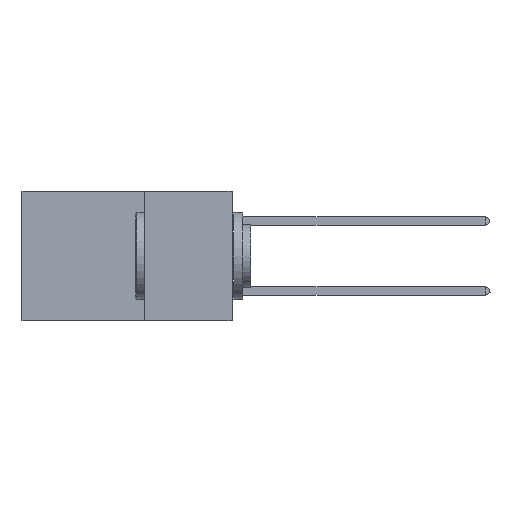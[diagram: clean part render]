
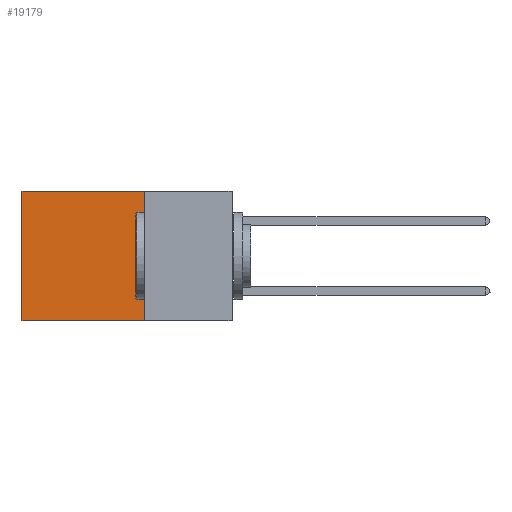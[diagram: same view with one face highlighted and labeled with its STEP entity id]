
A CAD part, left-side view. The second image highlights one B-rep face of the part: STEP entity #19179.
In plain terms, the highlighted planar face has unit normal (-1, 0, 0).
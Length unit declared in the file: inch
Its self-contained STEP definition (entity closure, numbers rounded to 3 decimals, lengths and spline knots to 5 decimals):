
#94 = LINE ( 'NONE', #131, #12554 ) ;
#131 = CARTESIAN_POINT ( 'NONE',  ( 0.2875, 0.25, -0.37 ) ) ;
#309 = VERTEX_POINT ( 'NONE', #5660 ) ;
#1466 = VERTEX_POINT ( 'NONE', #19495 ) ;
#2762 = CARTESIAN_POINT ( 'NONE',  ( 0.2875, 0.25, 0. ) ) ;
#2892 = VECTOR ( 'NONE', #17536, 39.37008 ) ;
#3384 = VERTEX_POINT ( 'NONE', #2762 ) ;
#4023 = CARTESIAN_POINT ( 'NONE',  ( 0.2875, 0.25, 0. ) ) ;
#4850 = CARTESIAN_POINT ( 'NONE',  ( 0.2875, 0.6, 0. ) ) ;
#5660 = CARTESIAN_POINT ( 'NONE',  ( 0.2875, 0.6, -0.37 ) ) ;
#6528 = CARTESIAN_POINT ( 'NONE',  ( 0.2875, 0.25, -0.37 ) ) ;
#7682 = DIRECTION ( 'NONE',  ( 1., 0., 0. ) ) ;
#7691 = AXIS2_PLACEMENT_3D ( 'NONE', #17827, #7682, #21393 ) ;
#7864 = ORIENTED_EDGE ( 'NONE', *, *, #19018, .F. ) ;
#8530 = VECTOR ( 'NONE', #10222, 39.37008 ) ;
#8904 = EDGE_CURVE ( 'NONE', #11808, #309, #94, .T. ) ;
#9281 = FACE_OUTER_BOUND ( 'NONE', #17351, .T. ) ;
#10222 = DIRECTION ( 'NONE',  ( 0., 0., -1. ) ) ;
#10639 = ORIENTED_EDGE ( 'NONE', *, *, #8904, .F. ) ;
#11808 = VERTEX_POINT ( 'NONE', #6528 ) ;
#12255 = ORIENTED_EDGE ( 'NONE', *, *, #18731, .T. ) ;
#12554 = VECTOR ( 'NONE', #18660, 39.37008 ) ;
#13443 = LINE ( 'NONE', #15403, #19291 ) ;
#13878 = ORIENTED_EDGE ( 'NONE', *, *, #14273, .T. ) ;
#14050 = LINE ( 'NONE', #4023, #2892 ) ;
#14273 = EDGE_CURVE ( 'NONE', #3384, #1466, #13443, .T. ) ;
#15403 = CARTESIAN_POINT ( 'NONE',  ( 0.2875, 0.25, 0. ) ) ;
#17100 = DIRECTION ( 'NONE',  ( 0., 1., 0. ) ) ;
#17351 = EDGE_LOOP ( 'NONE', ( #12255, #10639, #7864, #13878 ) ) ;
#17517 = LINE ( 'NONE', #4850, #8530 ) ;
#17536 = DIRECTION ( 'NONE',  ( 0., 0., -1. ) ) ;
#17827 = CARTESIAN_POINT ( 'NONE',  ( 0.2875, 0.25, 0. ) ) ;
#18052 = PLANE ( 'NONE',  #7691 ) ;
#18660 = DIRECTION ( 'NONE',  ( 0., 1., 0. ) ) ;
#18731 = EDGE_CURVE ( 'NONE', #1466, #309, #17517, .T. ) ;
#19018 = EDGE_CURVE ( 'NONE', #3384, #11808, #14050, .T. ) ;
#19179 = ADVANCED_FACE ( 'NONE', ( #9281 ), #18052, .F. ) ;
#19291 = VECTOR ( 'NONE', #17100, 39.37008 ) ;
#19495 = CARTESIAN_POINT ( 'NONE',  ( 0.2875, 0.6, 0. ) ) ;
#21393 = DIRECTION ( 'NONE',  ( 0., 0., -1. ) ) ;
